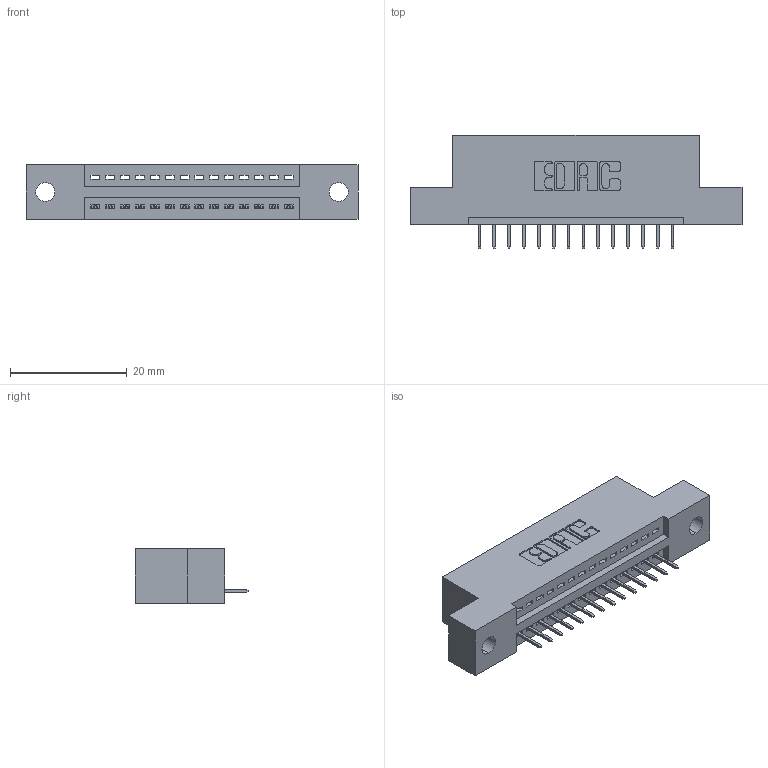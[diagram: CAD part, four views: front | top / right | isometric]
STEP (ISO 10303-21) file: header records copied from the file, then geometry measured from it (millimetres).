
FILE_DESCRIPTION (( 'STEP AP203' ), '1' );
FILE_NAME ('345-014-524-102.STEP', '2019-10-04T05:47:54', ( '' ), ( '' ), 'SwSTEP 2.0', 'SolidWorks 2016', '' );
FILE_SCHEMA (( 'CONFIG_CONTROL_DESIGN' ));
Length unit declared in the file: inch
Products named in the file (3): 345 Part_Flush Mounting Lugs - 0.128 Dia; 345-014-524-102; 345-292-001_345-293-124
Assembly tree (15 placements, depth 2):
  345-014-524-102
    345 Part_Flush Mounting Lugs - 0.128 Dia
    345-292-001_345-293-124  x14
Bounding box: 56.77 x 19.35 x 9.4 mm (x, y, z)
Volume: 5070.6 mm3; surface area: 5909.5 mm2
Topology: 15 solids, 15 shells, 994 faces, 2861 edges, 1850 vertices
Faces by surface type: plane 724, cylinder 270
Entity records: 14383 total; most frequent: CARTESIAN_POINT 2498, ORIENTED_EDGE 2446, DIRECTION 2223, EDGE_CURVE 1223, VECTOR 1039, LINE 1039, VERTEX_POINT 810, AXIS2_PLACEMENT_3D 592
